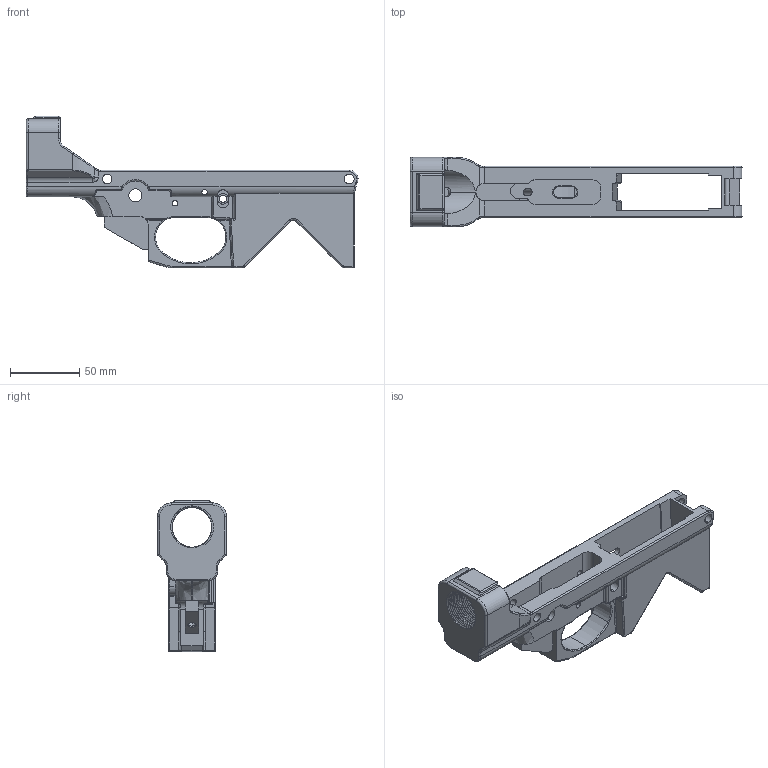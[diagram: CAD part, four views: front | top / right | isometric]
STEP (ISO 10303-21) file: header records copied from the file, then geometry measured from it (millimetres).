
FILE_DESCRIPTION (( 'STEP AP214' ), '1' );
FILE_NAME ('Abraxas_AR-10_V1.STEP', '2015-05-22T10:32:35', ( 'WarFairy' ), ( '' ), 'SwSTEP 2.0', 'SolidWorks 2015', '' );
FILE_SCHEMA (( 'AUTOMOTIVE_DESIGN' ));
Length unit declared in the file: inch
Products named in the file (1): Abraxas_AR-10_V1
Bounding box: 239.65 x 50 x 109.71 mm (x, y, z)
Volume: 209636.5 mm3; surface area: 69793.9 mm2
Topology: 1 solids, 1 shells, 502 faces, 1355 edges, 831 vertices
Faces by surface type: cylinder 228, plane 113, bspline 95, torus 54, cone 8, sphere 4
Entity records: 36041 total; most frequent: CARTESIAN_POINT 21048, ORIENTED_EDGE 2676, DIRECTION 2202, EDGE_CURVE 1338, VERTEX_POINT 831, AXIS2_PLACEMENT_3D 827, VECTOR 548, LINE 548
